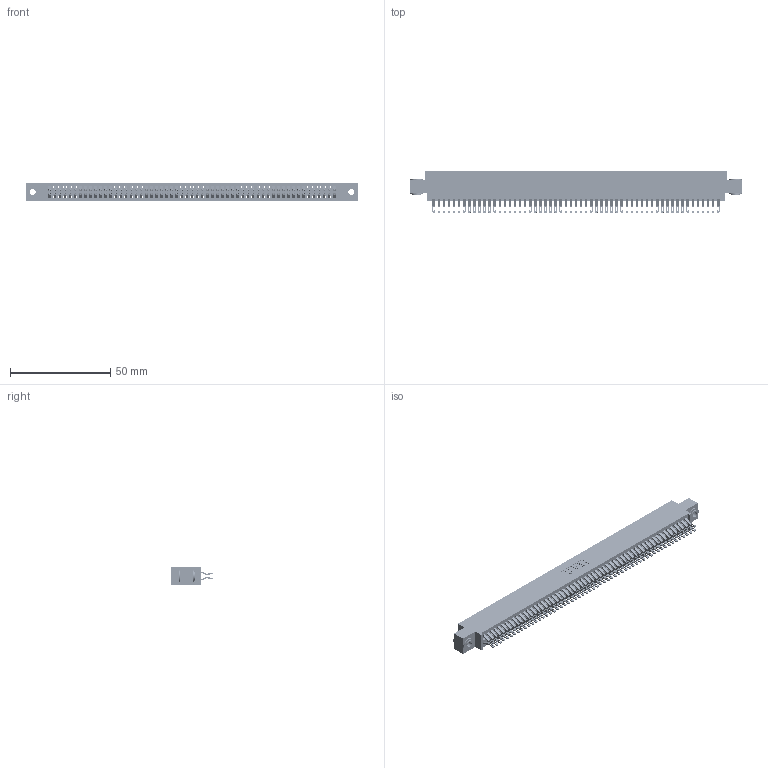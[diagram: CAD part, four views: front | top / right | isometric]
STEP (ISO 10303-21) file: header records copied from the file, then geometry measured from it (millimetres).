
FILE_DESCRIPTION (( 'STEP AP203' ), '1' );
FILE_NAME ('395-114-555-803.STEP', '2018-12-01T18:16:16', ( '' ), ( '' ), 'SwSTEP 2.0', 'SolidWorks 2016', '' );
FILE_SCHEMA (( 'CONFIG_CONTROL_DESIGN' ));
Length unit declared in the file: inch
Products named in the file (4): 395-114-555-803; 345 Part_0.170 Offset - 0.156 Dia-TH; 345-292-001_555 Tail; 345-250-002_345-250-002-102
Assembly tree (117 placements, depth 2):
  395-114-555-803
    345 Part_0.170 Offset - 0.156 Dia-TH
    345-292-001_555 Tail  x114
    345-250-002_345-250-002-102  x2
Bounding box: 165.99 x 21.13 x 9.4 mm (x, y, z)
Volume: 16500.2 mm3; surface area: 26179.1 mm2
Topology: 117 solids, 117 shells, 6552 faces, 20607 edges, 13734 vertices
Faces by surface type: plane 3628, cylinder 2916, cone 8
Entity records: 43812 total; most frequent: CARTESIAN_POINT 7341, ORIENTED_EDGE 7238, DIRECTION 6453, EDGE_CURVE 3619, VECTOR 3215, LINE 3215, VERTEX_POINT 2410, AXIS2_PLACEMENT_3D 1619
